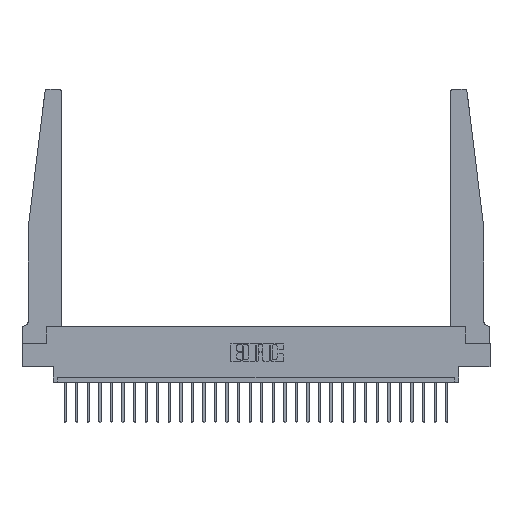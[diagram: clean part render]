
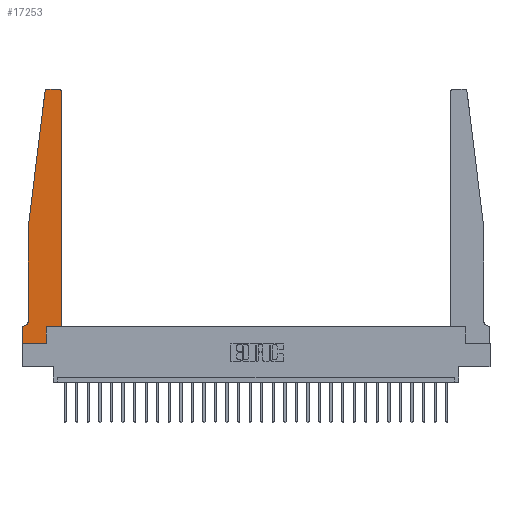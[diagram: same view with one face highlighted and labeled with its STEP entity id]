
A CAD part, top view. The second image highlights one B-rep face of the part: STEP entity #17253.
In plain terms, the highlighted planar face has unit normal (0, 0, 1).
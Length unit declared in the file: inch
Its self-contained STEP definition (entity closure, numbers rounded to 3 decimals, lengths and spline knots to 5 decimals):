
#791 = VERTEX_POINT ( 'NONE', #23308 ) ;
#912 = VERTEX_POINT ( 'NONE', #23988 ) ;
#1155 = CARTESIAN_POINT ( 'NONE',  ( 0., 0., 0.37 ) ) ;
#1361 = EDGE_CURVE ( 'NONE', #14761, #27236, #21310, .T. ) ;
#1400 = VECTOR ( 'NONE', #3477, 39.37008 ) ;
#1905 = CARTESIAN_POINT ( 'NONE',  ( 0.065, 1.25, 0.37 ) ) ;
#1913 = EDGE_CURVE ( 'NONE', #791, #10078, #26671, .T. ) ;
#2266 = CARTESIAN_POINT ( 'NONE',  ( 0.425, 0.18, 0.37 ) ) ;
#2823 = VECTOR ( 'NONE', #15169, 39.37008 ) ;
#2831 = CARTESIAN_POINT ( 'NONE',  ( 0.395, 2.72, 0.37 ) ) ;
#3174 = CARTESIAN_POINT ( 'NONE',  ( 0.2605, 0., 0.37 ) ) ;
#3223 = EDGE_LOOP ( 'NONE', ( #17297, #27057, #18606, #12707, #11456, #23507, #25638, #26039, #23135, #25485, #8148, #20734 ) ) ;
#3372 = CARTESIAN_POINT ( 'NONE',  ( 0., 0.1875, 0.37 ) ) ;
#3473 = VERTEX_POINT ( 'NONE', #16031 ) ;
#3477 = DIRECTION ( 'NONE',  ( -1., 0., 0. ) ) ;
#3648 = DIRECTION ( 'NONE',  ( 1., 0., 0. ) ) ;
#3792 = LINE ( 'NONE', #9405, #13005 ) ;
#4540 = VERTEX_POINT ( 'NONE', #23550 ) ;
#4584 = CARTESIAN_POINT ( 'NONE',  ( 0.2605, 0.18, 0.37 ) ) ;
#4793 = CARTESIAN_POINT ( 'NONE',  ( 0.015, 0.2375, 0.37 ) ) ;
#5092 = CARTESIAN_POINT ( 'NONE',  ( 0.395, 2.75, 0.37 ) ) ;
#5238 = CARTESIAN_POINT ( 'NONE',  ( 0.065, 1.25, 0.37 ) ) ;
#6770 = EDGE_CURVE ( 'NONE', #4540, #25300, #9224, .T. ) ;
#6812 = VERTEX_POINT ( 'NONE', #15779 ) ;
#7019 = CARTESIAN_POINT ( 'NONE',  ( 0., 0., 0.37 ) ) ;
#7177 = DIRECTION ( 'NONE',  ( 1., 0., 0. ) ) ;
#7765 = CARTESIAN_POINT ( 'NONE',  ( 0.425, 0.18, 0.37 ) ) ;
#8108 = VERTEX_POINT ( 'NONE', #3372 ) ;
#8148 = ORIENTED_EDGE ( 'NONE', *, *, #20513, .T. ) ;
#8185 = DIRECTION ( 'NONE',  ( 0., 0., 1. ) ) ;
#8676 = LINE ( 'NONE', #2266, #17386 ) ;
#9224 = CIRCLE ( 'NONE', #21681, 0.03 ) ;
#9225 = DIRECTION ( 'NONE',  ( 0., 0., -1. ) ) ;
#9405 = CARTESIAN_POINT ( 'NONE',  ( 0.425, 0.18, 0.37 ) ) ;
#9754 = CARTESIAN_POINT ( 'NONE',  ( 0.065, 0.1875, 0.37 ) ) ;
#10078 = VERTEX_POINT ( 'NONE', #3174 ) ;
#10148 = EDGE_CURVE ( 'NONE', #912, #6812, #16346, .T. ) ;
#11109 = DIRECTION ( 'NONE',  ( 0., 1., 0. ) ) ;
#11359 = EDGE_CURVE ( 'NONE', #8108, #791, #24138, .T. ) ;
#11373 = EDGE_CURVE ( 'NONE', #27236, #18898, #13709, .T. ) ;
#11456 = ORIENTED_EDGE ( 'NONE', *, *, #11373, .T. ) ;
#12194 = VECTOR ( 'NONE', #11109, 39.37008 ) ;
#12348 = LINE ( 'NONE', #1905, #2823 ) ;
#12707 = ORIENTED_EDGE ( 'NONE', *, *, #1361, .T. ) ;
#12872 = FACE_OUTER_BOUND ( 'NONE', #3223, .T. ) ;
#12882 = AXIS2_PLACEMENT_3D ( 'NONE', #21392, #18750, #23632 ) ;
#13005 = VECTOR ( 'NONE', #20805, 39.37008 ) ;
#13248 = DIRECTION ( 'NONE',  ( -1., 0., 0. ) ) ;
#13250 = VERTEX_POINT ( 'NONE', #7765 ) ;
#13709 = CIRCLE ( 'NONE', #14595, 0.05 ) ;
#14022 = CARTESIAN_POINT ( 'NONE',  ( 0.27653, 2.72, 0.37 ) ) ;
#14511 = CARTESIAN_POINT ( 'NONE',  ( 0.015, 0.1875, 0.37 ) ) ;
#14595 = AXIS2_PLACEMENT_3D ( 'NONE', #4793, #9225, #13248 ) ;
#14761 = VERTEX_POINT ( 'NONE', #5238 ) ;
#15169 = DIRECTION ( 'NONE',  ( -0.122, -0.992, 0. ) ) ;
#15776 = CARTESIAN_POINT ( 'NONE',  ( 0.25, 2.75, 0.37 ) ) ;
#15779 = CARTESIAN_POINT ( 'NONE',  ( 0.24675, 2.72367, 0.37 ) ) ;
#16031 = CARTESIAN_POINT ( 'NONE',  ( 0.2605, 0.18, 0.37 ) ) ;
#16346 = CIRCLE ( 'NONE', #25689, 0.03 ) ;
#16538 = DIRECTION ( 'NONE',  ( 1., 0., 0. ) ) ;
#17040 = DIRECTION ( 'NONE',  ( 1., 0., 0. ) ) ;
#17253 = ADVANCED_FACE ( 'NONE', ( #12872 ), #19033, .T. ) ;
#17297 = ORIENTED_EDGE ( 'NONE', *, *, #22269, .T. ) ;
#17386 = VECTOR ( 'NONE', #17040, 39.37008 ) ;
#17610 = LINE ( 'NONE', #15776, #25918 ) ;
#17887 = DIRECTION ( 'NONE',  ( -1., 0., 0. ) ) ;
#18606 = ORIENTED_EDGE ( 'NONE', *, *, #23332, .T. ) ;
#18750 = DIRECTION ( 'NONE',  ( 0., 0., 1. ) ) ;
#18817 = VECTOR ( 'NONE', #3648, 39.37008 ) ;
#18898 = VERTEX_POINT ( 'NONE', #14511 ) ;
#18925 = EDGE_CURVE ( 'NONE', #3473, #13250, #8676, .T. ) ;
#19033 = PLANE ( 'NONE',  #12882 ) ;
#20513 = EDGE_CURVE ( 'NONE', #13250, #4540, #3792, .T. ) ;
#20734 = ORIENTED_EDGE ( 'NONE', *, *, #6770, .T. ) ;
#20805 = DIRECTION ( 'NONE',  ( 0., 1., 0. ) ) ;
#21054 = EDGE_CURVE ( 'NONE', #18898, #8108, #24821, .T. ) ;
#21310 = LINE ( 'NONE', #24471, #25387 ) ;
#21392 = CARTESIAN_POINT ( 'NONE',  ( 0., 0.1875, 0.37 ) ) ;
#21430 = LINE ( 'NONE', #4584, #12194 ) ;
#21681 = AXIS2_PLACEMENT_3D ( 'NONE', #2831, #26530, #7177 ) ;
#22269 = EDGE_CURVE ( 'NONE', #25300, #912, #17610, .T. ) ;
#22780 = CARTESIAN_POINT ( 'NONE',  ( 0.065, 0.2375, 0.37 ) ) ;
#23135 = ORIENTED_EDGE ( 'NONE', *, *, #24761, .T. ) ;
#23308 = CARTESIAN_POINT ( 'NONE',  ( 0., 0., 0.37 ) ) ;
#23332 = EDGE_CURVE ( 'NONE', #6812, #14761, #12348, .T. ) ;
#23507 = ORIENTED_EDGE ( 'NONE', *, *, #21054, .T. ) ;
#23550 = CARTESIAN_POINT ( 'NONE',  ( 0.425, 2.72, 0.37 ) ) ;
#23554 = DIRECTION ( 'NONE',  ( 0., -1., 0. ) ) ;
#23632 = DIRECTION ( 'NONE',  ( 1., 0., 0. ) ) ;
#23988 = CARTESIAN_POINT ( 'NONE',  ( 0.27653, 2.75, 0.37 ) ) ;
#24004 = DIRECTION ( 'NONE',  ( 0., -1., 0. ) ) ;
#24138 = LINE ( 'NONE', #7019, #26654 ) ;
#24471 = CARTESIAN_POINT ( 'NONE',  ( 0.065, 1.25, 0.37 ) ) ;
#24761 = EDGE_CURVE ( 'NONE', #10078, #3473, #21430, .T. ) ;
#24821 = LINE ( 'NONE', #9754, #1400 ) ;
#25300 = VERTEX_POINT ( 'NONE', #5092 ) ;
#25387 = VECTOR ( 'NONE', #23554, 39.37008 ) ;
#25485 = ORIENTED_EDGE ( 'NONE', *, *, #18925, .T. ) ;
#25638 = ORIENTED_EDGE ( 'NONE', *, *, #11359, .T. ) ;
#25689 = AXIS2_PLACEMENT_3D ( 'NONE', #14022, #8185, #16538 ) ;
#25918 = VECTOR ( 'NONE', #17887, 39.37008 ) ;
#26039 = ORIENTED_EDGE ( 'NONE', *, *, #1913, .T. ) ;
#26530 = DIRECTION ( 'NONE',  ( 0., 0., 1. ) ) ;
#26654 = VECTOR ( 'NONE', #24004, 39.37008 ) ;
#26671 = LINE ( 'NONE', #1155, #18817 ) ;
#27057 = ORIENTED_EDGE ( 'NONE', *, *, #10148, .T. ) ;
#27236 = VERTEX_POINT ( 'NONE', #22780 ) ;
